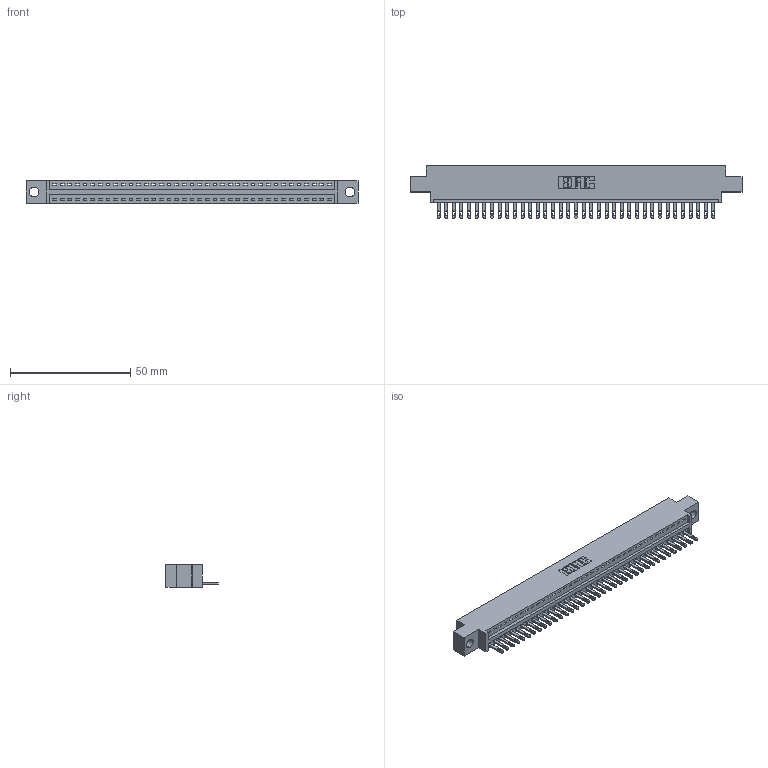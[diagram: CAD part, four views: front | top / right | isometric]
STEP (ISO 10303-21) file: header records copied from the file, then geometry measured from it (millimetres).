
FILE_DESCRIPTION (( 'STEP AP203' ), '1' );
FILE_NAME ('896-037-500-604.STEP', '2021-07-27T20:28:36', ( '' ), ( '' ), 'SwSTEP 2.0', 'SolidWorks 2020', '' );
FILE_SCHEMA (( 'CONFIG_CONTROL_DESIGN' ));
Length unit declared in the file: inch
Products named in the file (3): 345-292-001_345-293-100; 896-037-500-604; 846 Part_0.170 Offset - 0.156 Dia-TH
Assembly tree (38 placements, depth 2):
  896-037-500-604
    846 Part_0.170 Offset - 0.156 Dia-TH
    345-292-001_345-293-100  x37
Bounding box: 138.05 x 21.84 x 9.4 mm (x, y, z)
Volume: 12960.3 mm3; surface area: 16196.3 mm2
Topology: 38 solids, 38 shells, 2124 faces, 6557 edges, 4370 vertices
Faces by surface type: plane 1338, cylinder 786
Entity records: 23701 total; most frequent: CARTESIAN_POINT 4071, ORIENTED_EDGE 4042, DIRECTION 3599, EDGE_CURVE 2021, LINE 1737, VECTOR 1737, VERTEX_POINT 1346, AXIS2_PLACEMENT_3D 931
